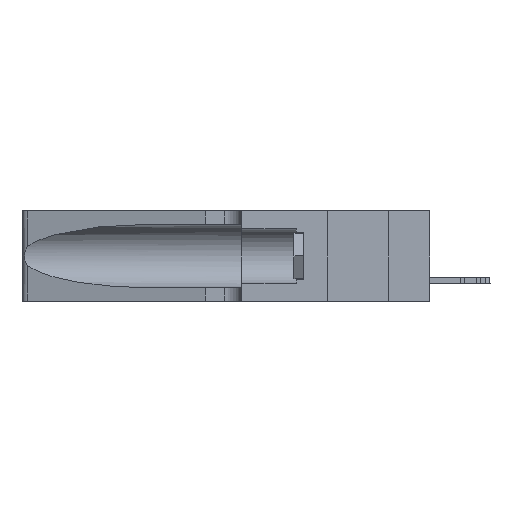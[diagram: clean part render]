
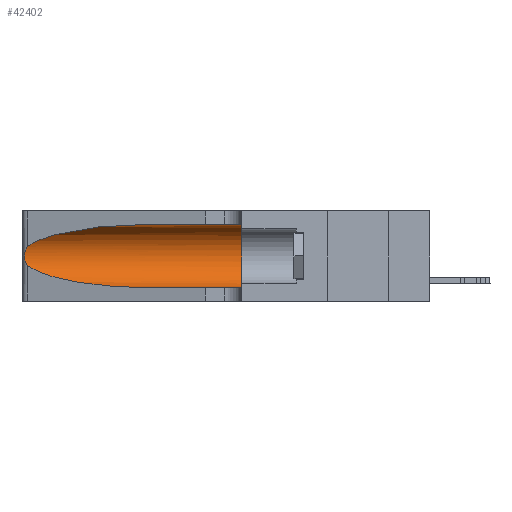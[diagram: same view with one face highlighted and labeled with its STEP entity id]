
A CAD part, left-side view. The second image highlights one B-rep face of the part: STEP entity #42402.
In plain terms, the highlighted cylindrical face has radius 3.308 mm (diameter 6.617 mm), a partial arc.
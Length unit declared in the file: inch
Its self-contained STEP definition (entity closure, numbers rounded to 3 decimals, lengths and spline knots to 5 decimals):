
#1934 = CARTESIAN_POINT ( 'NONE',  ( 0.18966, 0.96281, 0.05475 ) ) ;
#2273 = CARTESIAN_POINT ( 'NONE',  ( 0.25487, 1.22718, 0.22369 ) ) ;
#2831 =( BOUNDED_CURVE ( )  B_SPLINE_CURVE ( 3, ( #31731, #38990, #35118, #31021 ),
 .UNSPECIFIED., .F., .F. ) 
 B_SPLINE_CURVE_WITH_KNOTS ( ( 4, 4 ),
 ( 1.5708, 2.84003 ),
 .UNSPECIFIED. ) 
 CURVE ( )  GEOMETRIC_REPRESENTATION_ITEM ( )  RATIONAL_B_SPLINE_CURVE ( ( 1., 0.87, 0.87, 1. ) ) 
 REPRESENTATION_ITEM ( '' )  );
#3928 = VERTEX_POINT ( 'NONE', #21135 ) ;
#4251 = CARTESIAN_POINT ( 'NONE',  ( 0.25854, 1.2359, 0.20912 ) ) ;
#5798 = CARTESIAN_POINT ( 'NONE',  ( 0.1305, 1.61858, 0.31525 ) ) ;
#6059 = VERTEX_POINT ( 'NONE', #26219 ) ;
#8597 = VERTEX_POINT ( 'NONE', #50088 ) ;
#10425 = ORIENTED_EDGE ( 'NONE', *, *, #38344, .T. ) ;
#11177 = EDGE_CURVE ( 'NONE', #6059, #8597, #24547, .T. ) ;
#11647 = ORIENTED_EDGE ( 'NONE', *, *, #28144, .F. ) ;
#11673 = CARTESIAN_POINT ( 'NONE',  ( 0.26075, 1.23896, 0.19203 ) ) ;
#11851 = CARTESIAN_POINT ( 'NONE',  ( 0.25856, 1.23593, 0.16098 ) ) ;
#14090 = VERTEX_POINT ( 'NONE', #43896 ) ;
#14190 = CYLINDRICAL_SURFACE ( 'NONE', #44696, 0.13025 ) ;
#15063 = EDGE_CURVE ( 'NONE', #3928, #41226, #42431, .T. ) ;
#16841 = CARTESIAN_POINT ( 'NONE',  ( 0.1305, 0.35, 0.31525 ) ) ;
#16942 = CARTESIAN_POINT ( 'NONE',  ( 0.25487, 1.22718, 0.14631 ) ) ;
#17116 = EDGE_CURVE ( 'NONE', #3928, #6059, #2831, .T. ) ;
#18403 =( BOUNDED_CURVE ( )  B_SPLINE_CURVE ( 3, ( #37824, #22256, #1934, #30198 ),
 .UNSPECIFIED., .F., .F. ) 
 B_SPLINE_CURVE_WITH_KNOTS ( ( 4, 4 ),
 ( 3.44316, 4.71239 ),
 .UNSPECIFIED. ) 
 CURVE ( )  GEOMETRIC_REPRESENTATION_ITEM ( )  RATIONAL_B_SPLINE_CURVE ( ( 1., 0.87, 0.87, 1. ) ) 
 REPRESENTATION_ITEM ( '' )  );
#18960 = CARTESIAN_POINT ( 'NONE',  ( 0.1305, 0.35, 0.185 ) ) ;
#19005 = VERTEX_POINT ( 'NONE', #41600 ) ;
#19967 = CARTESIAN_POINT ( 'NONE',  ( 0.25639, 1.23186, 0.15144 ) ) ;
#21135 = CARTESIAN_POINT ( 'NONE',  ( 0.1305, 0.72297, 0.31525 ) ) ;
#22256 = CARTESIAN_POINT ( 'NONE',  ( 0.2373, 1.15595, 0.08982 ) ) ;
#23871 = CARTESIAN_POINT ( 'NONE',  ( 0.25787, 1.23484, 0.2124 ) ) ;
#24161 = DIRECTION ( 'NONE',  ( 0., -1., 0. ) ) ;
#24547 = B_SPLINE_CURVE_WITH_KNOTS ( 'NONE', 3,
 ( #2273, #52298, #35939, #23871, #4251, #44389, #11673, #44046, #52117, #11851, #44219, #19967, #28084, #16942 ),
 .UNSPECIFIED., .F., .F.,
 ( 4, 2, 2, 2, 2, 2, 4 ),
 ( 0., 0.00027, 0.00053, 0.00107, 0.0016, 0.00187, 0.00214 ),
 .UNSPECIFIED. ) ;
#26219 = CARTESIAN_POINT ( 'NONE',  ( 0.25487, 1.22718, 0.22369 ) ) ;
#28084 = CARTESIAN_POINT ( 'NONE',  ( 0.25555, 1.22993, 0.14849 ) ) ;
#28144 = EDGE_CURVE ( 'NONE', #41226, #14090, #40474, .T. ) ;
#30198 = CARTESIAN_POINT ( 'NONE',  ( 0.1305, 0.72297, 0.05475 ) ) ;
#31021 = CARTESIAN_POINT ( 'NONE',  ( 0.25487, 1.22718, 0.22369 ) ) ;
#31183 = ORIENTED_EDGE ( 'NONE', *, *, #17116, .T. ) ;
#31186 = CARTESIAN_POINT ( 'NONE',  ( 0.1305, 1.61858, 0.05475 ) ) ;
#31731 = CARTESIAN_POINT ( 'NONE',  ( 0.1305, 0.72297, 0.31525 ) ) ;
#33899 = LINE ( 'NONE', #31186, #49018 ) ;
#35118 = CARTESIAN_POINT ( 'NONE',  ( 0.2373, 1.15595, 0.28018 ) ) ;
#35247 = ORIENTED_EDGE ( 'NONE', *, *, #11177, .T. ) ;
#35257 = DIRECTION ( 'NONE',  ( 0., 1., 0. ) ) ;
#35885 = DIRECTION ( 'NONE',  ( 0., 0., -1. ) ) ;
#35939 = CARTESIAN_POINT ( 'NONE',  ( 0.25639, 1.23184, 0.21858 ) ) ;
#36223 = CARTESIAN_POINT ( 'NONE',  ( 0.1305, 1.61858, 0.185 ) ) ;
#37824 = CARTESIAN_POINT ( 'NONE',  ( 0.25487, 1.22718, 0.14631 ) ) ;
#38344 = EDGE_CURVE ( 'NONE', #8597, #19005, #18403, .T. ) ;
#38990 = CARTESIAN_POINT ( 'NONE',  ( 0.18966, 0.96281, 0.31525 ) ) ;
#39133 = EDGE_CURVE ( 'NONE', #19005, #14090, #33899, .T. ) ;
#39393 = ORIENTED_EDGE ( 'NONE', *, *, #39133, .T. ) ;
#40474 = CIRCLE ( 'NONE', #45774, 0.13025 ) ;
#41226 = VERTEX_POINT ( 'NONE', #16841 ) ;
#41600 = CARTESIAN_POINT ( 'NONE',  ( 0.1305, 0.72297, 0.05475 ) ) ;
#42402 = ADVANCED_FACE ( 'NONE', ( #43952 ), #14190, .F. ) ;
#42431 = LINE ( 'NONE', #5798, #45535 ) ;
#43378 = DIRECTION ( 'NONE',  ( 0., 0., 1. ) ) ;
#43896 = CARTESIAN_POINT ( 'NONE',  ( 0.1305, 0.35, 0.05475 ) ) ;
#43952 = FACE_OUTER_BOUND ( 'NONE', #45911, .T. ) ;
#44046 = CARTESIAN_POINT ( 'NONE',  ( 0.26075, 1.23896, 0.178 ) ) ;
#44219 = CARTESIAN_POINT ( 'NONE',  ( 0.25789, 1.23486, 0.15765 ) ) ;
#44389 = CARTESIAN_POINT ( 'NONE',  ( 0.26018, 1.23835, 0.19895 ) ) ;
#44696 = AXIS2_PLACEMENT_3D ( 'NONE', #36223, #24161, #35885 ) ;
#45535 = VECTOR ( 'NONE', #45898, 39.37008 ) ;
#45774 = AXIS2_PLACEMENT_3D ( 'NONE', #18960, #35257, #43378 ) ;
#45898 = DIRECTION ( 'NONE',  ( 0., -1., 0. ) ) ;
#45911 = EDGE_LOOP ( 'NONE', ( #31183, #35247, #10425, #39393, #11647, #47480 ) ) ;
#47480 = ORIENTED_EDGE ( 'NONE', *, *, #15063, .F. ) ;
#49018 = VECTOR ( 'NONE', #50956, 39.37008 ) ;
#50088 = CARTESIAN_POINT ( 'NONE',  ( 0.25487, 1.22718, 0.14631 ) ) ;
#50956 = DIRECTION ( 'NONE',  ( 0., -1., 0. ) ) ;
#52117 = CARTESIAN_POINT ( 'NONE',  ( 0.26017, 1.23833, 0.17102 ) ) ;
#52298 = CARTESIAN_POINT ( 'NONE',  ( 0.25555, 1.22994, 0.2215 ) ) ;
